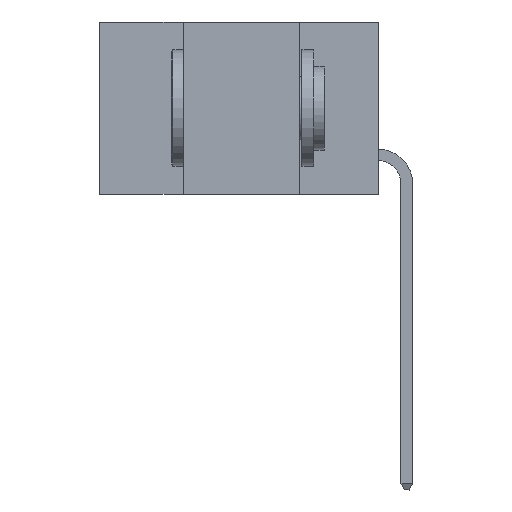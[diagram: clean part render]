
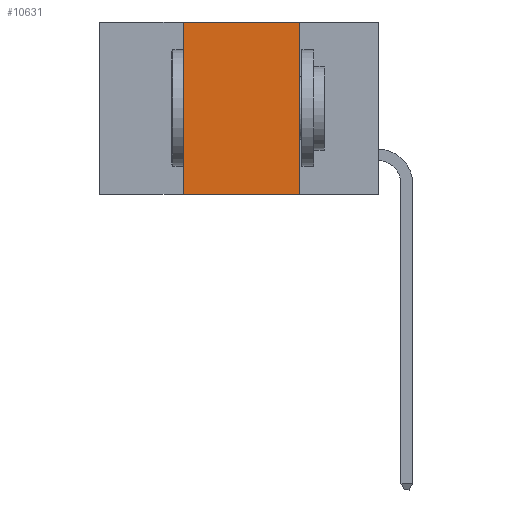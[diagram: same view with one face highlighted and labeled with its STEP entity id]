
A CAD part, left-side view. The second image highlights one B-rep face of the part: STEP entity #10631.
In plain terms, the highlighted planar face has unit normal (-1, 0, 0).
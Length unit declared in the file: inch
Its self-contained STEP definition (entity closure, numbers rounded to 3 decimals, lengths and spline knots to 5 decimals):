
#36 = VERTEX_POINT ( 'NONE', #1332 ) ;
#968 = EDGE_CURVE ( 'NONE', #36, #16289, #12408, .T. ) ;
#1332 = CARTESIAN_POINT ( 'NONE',  ( 0., 0.42, -0.37 ) ) ;
#1424 = EDGE_CURVE ( 'NONE', #10580, #3847, #12019, .T. ) ;
#1441 = AXIS2_PLACEMENT_3D ( 'NONE', #5434, #6800, #15692 ) ;
#1812 = VECTOR ( 'NONE', #12740, 39.37008 ) ;
#1970 = DIRECTION ( 'NONE',  ( 0., 0., -1. ) ) ;
#2528 = DIRECTION ( 'NONE',  ( 0., 0., 1. ) ) ;
#2591 = LINE ( 'NONE', #12064, #5753 ) ;
#2762 = EDGE_CURVE ( 'NONE', #36, #10580, #3031, .T. ) ;
#3031 = LINE ( 'NONE', #4561, #6235 ) ;
#3583 = CARTESIAN_POINT ( 'NONE',  ( 0., 0.6, -0.37 ) ) ;
#3637 = ORIENTED_EDGE ( 'NONE', *, *, #2762, .F. ) ;
#3639 = DIRECTION ( 'NONE',  ( 0., -1., 0. ) ) ;
#3680 = EDGE_CURVE ( 'NONE', #3847, #16289, #2591, .T. ) ;
#3779 = CARTESIAN_POINT ( 'NONE',  ( 0., 0.17, -0.37 ) ) ;
#3847 = VERTEX_POINT ( 'NONE', #12001 ) ;
#4561 = CARTESIAN_POINT ( 'NONE',  ( 0., 0.42, 0. ) ) ;
#5320 = CARTESIAN_POINT ( 'NONE',  ( 0., 0.42, 0. ) ) ;
#5434 = CARTESIAN_POINT ( 'NONE',  ( 0., 0.6, 0. ) ) ;
#5753 = VECTOR ( 'NONE', #1970, 39.37008 ) ;
#6235 = VECTOR ( 'NONE', #2528, 39.37008 ) ;
#6800 = DIRECTION ( 'NONE',  ( 1., 0., 0. ) ) ;
#7214 = ORIENTED_EDGE ( 'NONE', *, *, #968, .T. ) ;
#7285 = CARTESIAN_POINT ( 'NONE',  ( 0., 0.6, 0. ) ) ;
#10332 = ORIENTED_EDGE ( 'NONE', *, *, #1424, .F. ) ;
#10580 = VERTEX_POINT ( 'NONE', #5320 ) ;
#10631 = ADVANCED_FACE ( 'NONE', ( #10961 ), #13245, .F. ) ;
#10961 = FACE_OUTER_BOUND ( 'NONE', #13998, .T. ) ;
#12001 = CARTESIAN_POINT ( 'NONE',  ( 0., 0.17, 0. ) ) ;
#12019 = LINE ( 'NONE', #7285, #1812 ) ;
#12064 = CARTESIAN_POINT ( 'NONE',  ( 0., 0.17, 0. ) ) ;
#12408 = LINE ( 'NONE', #3583, #12816 ) ;
#12740 = DIRECTION ( 'NONE',  ( 0., -1., 0. ) ) ;
#12816 = VECTOR ( 'NONE', #3639, 39.37008 ) ;
#13245 = PLANE ( 'NONE',  #1441 ) ;
#13998 = EDGE_LOOP ( 'NONE', ( #16515, #10332, #3637, #7214 ) ) ;
#15692 = DIRECTION ( 'NONE',  ( 0., 0., -1. ) ) ;
#16289 = VERTEX_POINT ( 'NONE', #3779 ) ;
#16515 = ORIENTED_EDGE ( 'NONE', *, *, #3680, .F. ) ;
